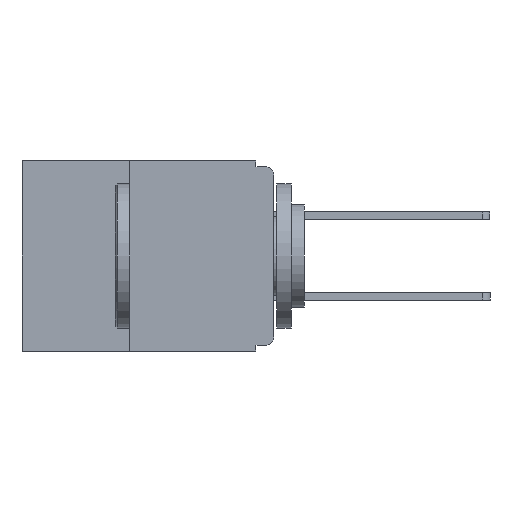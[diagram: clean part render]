
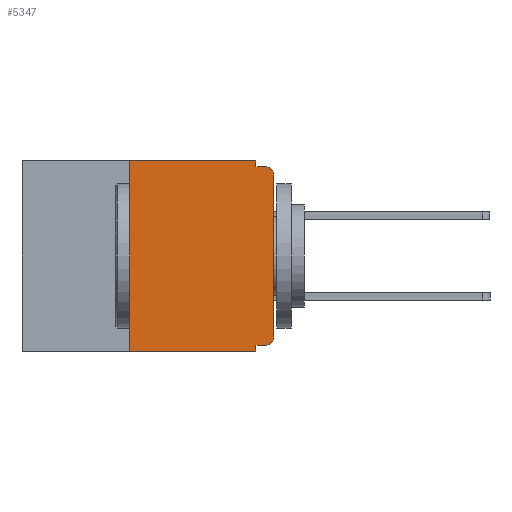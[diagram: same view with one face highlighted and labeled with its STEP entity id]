
A CAD part, left-side view. The second image highlights one B-rep face of the part: STEP entity #5347.
In plain terms, the highlighted planar face has unit normal (-1, 0, 0).
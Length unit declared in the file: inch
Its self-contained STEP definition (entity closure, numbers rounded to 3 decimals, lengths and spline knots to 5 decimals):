
#106 = VECTOR ( 'NONE', #16014, 39.37008 ) ;
#563 = CARTESIAN_POINT ( 'NONE',  ( 0., 0.437, -0.33 ) ) ;
#921 = EDGE_CURVE ( 'NONE', #5517, #3398, #9121, .T. ) ;
#972 = VERTEX_POINT ( 'NONE', #15397 ) ;
#1510 = CARTESIAN_POINT ( 'NONE',  ( 0., 0.25, 0. ) ) ;
#1521 = CARTESIAN_POINT ( 'NONE',  ( 0., 0.031, -0.01 ) ) ;
#1532 = FACE_OUTER_BOUND ( 'NONE', #2746, .T. ) ;
#2083 = EDGE_CURVE ( 'NONE', #9873, #16568, #14686, .T. ) ;
#2265 = DIRECTION ( 'NONE',  ( 0., -1., 0. ) ) ;
#2566 = ORIENTED_EDGE ( 'NONE', *, *, #9478, .T. ) ;
#2645 = VECTOR ( 'NONE', #7317, 39.37008 ) ;
#2705 = ORIENTED_EDGE ( 'NONE', *, *, #12904, .T. ) ;
#2746 = EDGE_LOOP ( 'NONE', ( #2566, #2705, #3243, #3490, #3596, #3617, #3702, #4084, #4404, #4535 ) ) ;
#3138 = LINE ( 'NONE', #7360, #2645 ) ;
#3243 = ORIENTED_EDGE ( 'NONE', *, *, #2083, .F. ) ;
#3369 = LINE ( 'NONE', #15865, #4412 ) ;
#3398 = VERTEX_POINT ( 'NONE', #6359 ) ;
#3490 = ORIENTED_EDGE ( 'NONE', *, *, #14958, .F. ) ;
#3596 = ORIENTED_EDGE ( 'NONE', *, *, #921, .F. ) ;
#3617 = ORIENTED_EDGE ( 'NONE', *, *, #13977, .F. ) ;
#3702 = ORIENTED_EDGE ( 'NONE', *, *, #13021, .T. ) ;
#3710 = AXIS2_PLACEMENT_3D ( 'NONE', #18357, #18324, #18298 ) ;
#3743 = AXIS2_PLACEMENT_3D ( 'NONE', #17122, #8327, #18494 ) ;
#4084 = ORIENTED_EDGE ( 'NONE', *, *, #12005, .F. ) ;
#4404 = ORIENTED_EDGE ( 'NONE', *, *, #16741, .F. ) ;
#4412 = VECTOR ( 'NONE', #5388, 39.37008 ) ;
#4484 = AXIS2_PLACEMENT_3D ( 'NONE', #12261, #12212, #12006 ) ;
#4535 = ORIENTED_EDGE ( 'NONE', *, *, #10848, .T. ) ;
#4645 = VERTEX_POINT ( 'NONE', #18286 ) ;
#4903 = LINE ( 'NONE', #7869, #16390 ) ;
#5347 = ADVANCED_FACE ( 'NONE', ( #1532 ), #12230, .F. ) ;
#5388 = DIRECTION ( 'NONE',  ( 0., 1., 0. ) ) ;
#5517 = VERTEX_POINT ( 'NONE', #1510 ) ;
#5987 = DIRECTION ( 'NONE',  ( 0., 0., -1. ) ) ;
#6264 = DIRECTION ( 'NONE',  ( 0., -1., 0. ) ) ;
#6284 = CARTESIAN_POINT ( 'NONE',  ( 0., 0., -0.01 ) ) ;
#6359 = CARTESIAN_POINT ( 'NONE',  ( 0., 0.031, 0. ) ) ;
#7317 = DIRECTION ( 'NONE',  ( 0., 0., 1. ) ) ;
#7360 = CARTESIAN_POINT ( 'NONE',  ( 0., 0., 0. ) ) ;
#7384 = VECTOR ( 'NONE', #2265, 39.37008 ) ;
#7467 = CARTESIAN_POINT ( 'NONE',  ( 0., 0.031, -0.33 ) ) ;
#7509 = CARTESIAN_POINT ( 'NONE',  ( 0., 0.031, 0. ) ) ;
#7822 = DIRECTION ( 'NONE',  ( 0., 0., -1. ) ) ;
#7869 = CARTESIAN_POINT ( 'NONE',  ( 0., 0.25, -0.33 ) ) ;
#8193 = CIRCLE ( 'NONE', #3710, 0.015 ) ;
#8327 = DIRECTION ( 'NONE',  ( -1., 0., 0. ) ) ;
#8386 = LINE ( 'NONE', #7467, #19477 ) ;
#9121 = LINE ( 'NONE', #10338, #106 ) ;
#9478 = EDGE_CURVE ( 'NONE', #11697, #11010, #3138, .T. ) ;
#9873 = VERTEX_POINT ( 'NONE', #1521 ) ;
#10124 = CARTESIAN_POINT ( 'NONE',  ( 0., 0.031, -0.32 ) ) ;
#10338 = CARTESIAN_POINT ( 'NONE',  ( 0., 0.437, 0. ) ) ;
#10610 = CARTESIAN_POINT ( 'NONE',  ( 0., 0., -0.305 ) ) ;
#10719 = VECTOR ( 'NONE', #6264, 39.37008 ) ;
#10848 = EDGE_CURVE ( 'NONE', #4645, #11697, #8193, .T. ) ;
#11010 = VERTEX_POINT ( 'NONE', #16894 ) ;
#11697 = VERTEX_POINT ( 'NONE', #10610 ) ;
#12005 = EDGE_CURVE ( 'NONE', #13701, #18963, #8386, .T. ) ;
#12006 = DIRECTION ( 'NONE',  ( 0., 0., -1. ) ) ;
#12088 = CARTESIAN_POINT ( 'NONE',  ( 0., 0.031, -0.33 ) ) ;
#12212 = DIRECTION ( 'NONE',  ( 1., 0., 0. ) ) ;
#12230 = PLANE ( 'NONE',  #4484 ) ;
#12261 = CARTESIAN_POINT ( 'NONE',  ( 0., 0.437, 0. ) ) ;
#12904 = EDGE_CURVE ( 'NONE', #11010, #16568, #17084, .T. ) ;
#13021 = EDGE_CURVE ( 'NONE', #972, #18963, #15330, .T. ) ;
#13701 = VERTEX_POINT ( 'NONE', #10124 ) ;
#13977 = EDGE_CURVE ( 'NONE', #972, #5517, #4903, .T. ) ;
#13982 = CARTESIAN_POINT ( 'NONE',  ( 0., 0.015, -0.01 ) ) ;
#14104 = VECTOR ( 'NONE', #5987, 39.37008 ) ;
#14686 = LINE ( 'NONE', #6284, #10719 ) ;
#14958 = EDGE_CURVE ( 'NONE', #3398, #9873, #15906, .T. ) ;
#15315 = DIRECTION ( 'NONE',  ( 0., 0., 1. ) ) ;
#15330 = LINE ( 'NONE', #563, #7384 ) ;
#15397 = CARTESIAN_POINT ( 'NONE',  ( 0., 0.25, -0.33 ) ) ;
#15865 = CARTESIAN_POINT ( 'NONE',  ( 0., 0., -0.32 ) ) ;
#15906 = LINE ( 'NONE', #7509, #14104 ) ;
#16014 = DIRECTION ( 'NONE',  ( 0., -1., 0. ) ) ;
#16390 = VECTOR ( 'NONE', #15315, 39.37008 ) ;
#16568 = VERTEX_POINT ( 'NONE', #13982 ) ;
#16741 = EDGE_CURVE ( 'NONE', #4645, #13701, #3369, .T. ) ;
#16894 = CARTESIAN_POINT ( 'NONE',  ( 0., 0., -0.025 ) ) ;
#17084 = CIRCLE ( 'NONE', #3743, 0.015 ) ;
#17122 = CARTESIAN_POINT ( 'NONE',  ( 0., 0.015, -0.025 ) ) ;
#18286 = CARTESIAN_POINT ( 'NONE',  ( 0., 0.015, -0.32 ) ) ;
#18298 = DIRECTION ( 'NONE',  ( 0., 0., -1. ) ) ;
#18324 = DIRECTION ( 'NONE',  ( -1., 0., 0. ) ) ;
#18357 = CARTESIAN_POINT ( 'NONE',  ( 0., 0.015, -0.305 ) ) ;
#18494 = DIRECTION ( 'NONE',  ( 0., 0., -1. ) ) ;
#18963 = VERTEX_POINT ( 'NONE', #12088 ) ;
#19477 = VECTOR ( 'NONE', #7822, 39.37008 ) ;
